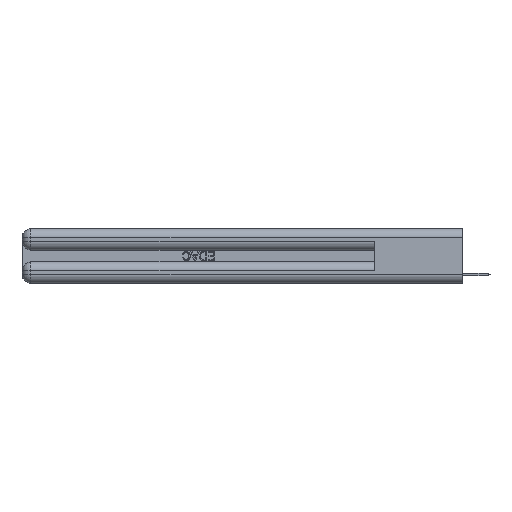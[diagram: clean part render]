
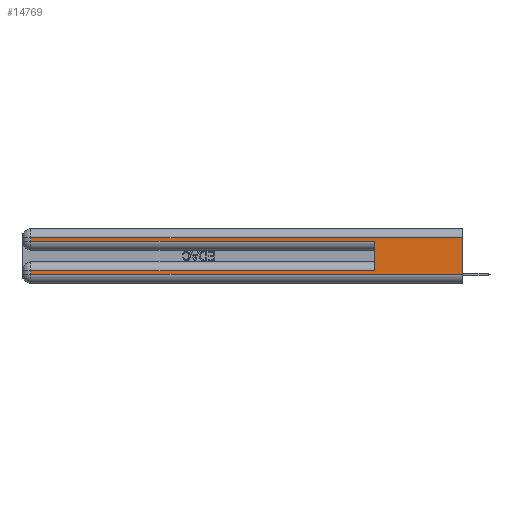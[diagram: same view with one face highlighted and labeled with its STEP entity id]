
A CAD part, left-side view. The second image highlights one B-rep face of the part: STEP entity #14769.
In plain terms, the highlighted planar face has unit normal (-1, 0, 0).
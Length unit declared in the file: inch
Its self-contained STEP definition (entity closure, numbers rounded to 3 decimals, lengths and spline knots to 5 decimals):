
#2334 = ORIENTED_EDGE ( 'NONE', *, *, #24721, .T. ) ;
#2671 = VERTEX_POINT ( 'NONE', #22993 ) ;
#3234 = ORIENTED_EDGE ( 'NONE', *, *, #6477, .T. ) ;
#3637 = EDGE_CURVE ( 'NONE', #18085, #5358, #22407, .T. ) ;
#3862 = ORIENTED_EDGE ( 'NONE', *, *, #18329, .F. ) ;
#3999 = ORIENTED_EDGE ( 'NONE', *, *, #25384, .T. ) ;
#4044 = CARTESIAN_POINT ( 'NONE',  ( 0., 2.94, 0.06 ) ) ;
#4459 = EDGE_LOOP ( 'NONE', ( #20755, #2334, #14807, #3234, #3862, #18803, #3999, #26595 ) ) ;
#4708 = CARTESIAN_POINT ( 'NONE',  ( 0., 0.6, 0.145 ) ) ;
#4737 = DIRECTION ( 'NONE',  ( 0., 1., 0. ) ) ;
#4821 = CARTESIAN_POINT ( 'NONE',  ( 0., 2.94, 0.285 ) ) ;
#4908 = CARTESIAN_POINT ( 'NONE',  ( 0., 0., 0.085 ) ) ;
#5234 = VERTEX_POINT ( 'NONE', #4821 ) ;
#5358 = VERTEX_POINT ( 'NONE', #18467 ) ;
#5601 = VERTEX_POINT ( 'NONE', #21039 ) ;
#5671 = LINE ( 'NONE', #15911, #32196 ) ;
#5677 = CARTESIAN_POINT ( 'NONE',  ( 0., 2.94, 0.31 ) ) ;
#6477 = EDGE_CURVE ( 'NONE', #5234, #5601, #14563, .T. ) ;
#6603 = PLANE ( 'NONE',  #24198 ) ;
#7483 = VECTOR ( 'NONE', #28774, 39.37008 ) ;
#7714 = CARTESIAN_POINT ( 'NONE',  ( 0., 2.94, 0.37 ) ) ;
#8028 = CARTESIAN_POINT ( 'NONE',  ( 0., 2.94, 0.085 ) ) ;
#8561 = VERTEX_POINT ( 'NONE', #5677 ) ;
#9148 = DIRECTION ( 'NONE',  ( 0., -1., 0. ) ) ;
#9487 = VECTOR ( 'NONE', #11726, 39.37008 ) ;
#10213 = DIRECTION ( 'NONE',  ( 0., 0., -1. ) ) ;
#11726 = DIRECTION ( 'NONE',  ( 0., -1., 0. ) ) ;
#11770 = VECTOR ( 'NONE', #10213, 39.37008 ) ;
#11883 = CARTESIAN_POINT ( 'NONE',  ( 0., 0., 0.285 ) ) ;
#12459 = VECTOR ( 'NONE', #9148, 39.37008 ) ;
#14563 = LINE ( 'NONE', #11883, #9487 ) ;
#14769 = ADVANCED_FACE ( 'NONE', ( #16376 ), #6603, .F. ) ;
#14807 = ORIENTED_EDGE ( 'NONE', *, *, #18004, .T. ) ;
#15477 = LINE ( 'NONE', #4708, #26841 ) ;
#15911 = CARTESIAN_POINT ( 'NONE',  ( 0., 0., 0.37 ) ) ;
#16376 = FACE_OUTER_BOUND ( 'NONE', #4459, .T. ) ;
#17073 = CARTESIAN_POINT ( 'NONE',  ( 0., 0., 0.31 ) ) ;
#17224 = VERTEX_POINT ( 'NONE', #8028 ) ;
#18004 = EDGE_CURVE ( 'NONE', #8561, #5234, #24063, .T. ) ;
#18085 = VERTEX_POINT ( 'NONE', #4044 ) ;
#18329 = EDGE_CURVE ( 'NONE', #2671, #5601, #15477, .T. ) ;
#18467 = CARTESIAN_POINT ( 'NONE',  ( 0., 0., 0.06 ) ) ;
#18562 = CARTESIAN_POINT ( 'NONE',  ( 0., 2.94, 0.37 ) ) ;
#18803 = ORIENTED_EDGE ( 'NONE', *, *, #27584, .T. ) ;
#19213 = CARTESIAN_POINT ( 'NONE',  ( 0., 0., 0.31 ) ) ;
#19765 = VECTOR ( 'NONE', #28944, 39.37008 ) ;
#20755 = ORIENTED_EDGE ( 'NONE', *, *, #25865, .F. ) ;
#21039 = CARTESIAN_POINT ( 'NONE',  ( 0., 0.6, 0.285 ) ) ;
#21409 = DIRECTION ( 'NONE',  ( 1., 0., 0. ) ) ;
#22056 = DIRECTION ( 'NONE',  ( 0., 0., -1. ) ) ;
#22074 = LINE ( 'NONE', #4908, #31871 ) ;
#22407 = LINE ( 'NONE', #32655, #12459 ) ;
#22993 = CARTESIAN_POINT ( 'NONE',  ( 0., 0.6, 0.085 ) ) ;
#23868 = VERTEX_POINT ( 'NONE', #17073 ) ;
#24063 = LINE ( 'NONE', #18562, #7483 ) ;
#24077 = CARTESIAN_POINT ( 'NONE',  ( 0., 0., 0.37 ) ) ;
#24198 = AXIS2_PLACEMENT_3D ( 'NONE', #24077, #21409, #22056 ) ;
#24721 = EDGE_CURVE ( 'NONE', #23868, #8561, #31487, .T. ) ;
#25384 = EDGE_CURVE ( 'NONE', #17224, #18085, #33067, .T. ) ;
#25865 = EDGE_CURVE ( 'NONE', #23868, #5358, #5671, .T. ) ;
#26595 = ORIENTED_EDGE ( 'NONE', *, *, #3637, .T. ) ;
#26841 = VECTOR ( 'NONE', #32945, 39.37008 ) ;
#27584 = EDGE_CURVE ( 'NONE', #2671, #17224, #22074, .T. ) ;
#28774 = DIRECTION ( 'NONE',  ( 0., 0., -1. ) ) ;
#28944 = DIRECTION ( 'NONE',  ( 0., 1., 0. ) ) ;
#30855 = DIRECTION ( 'NONE',  ( 0., 0., -1. ) ) ;
#31487 = LINE ( 'NONE', #19213, #19765 ) ;
#31871 = VECTOR ( 'NONE', #4737, 39.37008 ) ;
#32196 = VECTOR ( 'NONE', #30855, 39.37008 ) ;
#32655 = CARTESIAN_POINT ( 'NONE',  ( 0., 0., 0.06 ) ) ;
#32945 = DIRECTION ( 'NONE',  ( 0., 0., 1. ) ) ;
#33067 = LINE ( 'NONE', #7714, #11770 ) ;
